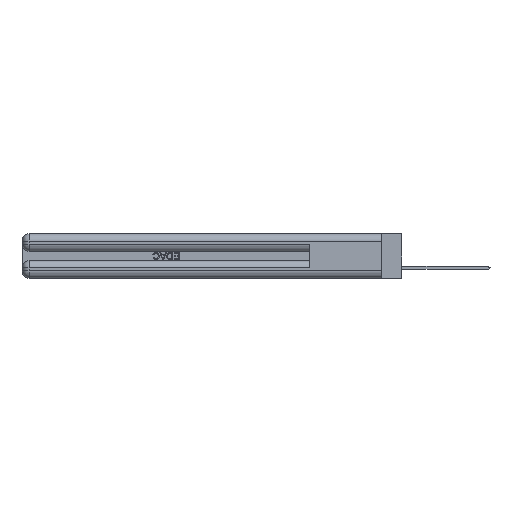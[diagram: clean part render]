
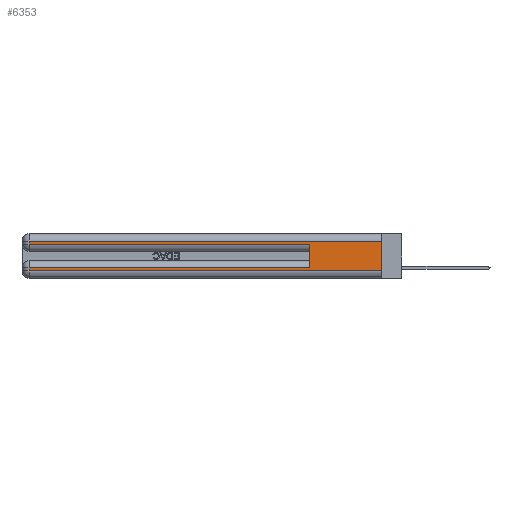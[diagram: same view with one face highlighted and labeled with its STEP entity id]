
A CAD part, left-side view. The second image highlights one B-rep face of the part: STEP entity #6353.
In plain terms, the highlighted planar face has unit normal (-1, 0, 0).
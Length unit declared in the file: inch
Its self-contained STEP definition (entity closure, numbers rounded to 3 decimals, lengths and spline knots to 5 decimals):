
#823 = LINE ( 'NONE', #51536, #43742 ) ;
#1345 = VECTOR ( 'NONE', #28418, 39.37008 ) ;
#1514 = CARTESIAN_POINT ( 'NONE',  ( 0., 0.6, 0.085 ) ) ;
#2061 = AXIS2_PLACEMENT_3D ( 'NONE', #14493, #38792, #19449 ) ;
#2967 = VERTEX_POINT ( 'NONE', #52110 ) ;
#2993 = ORIENTED_EDGE ( 'NONE', *, *, #46046, .T. ) ;
#3393 = CARTESIAN_POINT ( 'NONE',  ( 0., 2.94, 0.37 ) ) ;
#4040 = DIRECTION ( 'NONE',  ( 0., 0., -1. ) ) ;
#4673 = EDGE_LOOP ( 'NONE', ( #17953, #2993, #53097, #30266, #6761, #10194, #51034, #38221 ) ) ;
#4704 = VECTOR ( 'NONE', #52889, 39.37008 ) ;
#4742 = LINE ( 'NONE', #49902, #22289 ) ;
#6000 = DIRECTION ( 'NONE',  ( 0., 1., 0. ) ) ;
#6353 = ADVANCED_FACE ( 'NONE', ( #23500 ), #45315, .F. ) ;
#6634 = VERTEX_POINT ( 'NONE', #34424 ) ;
#6761 = ORIENTED_EDGE ( 'NONE', *, *, #43200, .F. ) ;
#7972 = VECTOR ( 'NONE', #41180, 39.37008 ) ;
#8007 = CARTESIAN_POINT ( 'NONE',  ( 0., 2.94, 0.37 ) ) ;
#8946 = LINE ( 'NONE', #8007, #40845 ) ;
#9210 = CARTESIAN_POINT ( 'NONE',  ( 0., 0., 0.31 ) ) ;
#9835 = EDGE_CURVE ( 'NONE', #46352, #6634, #4742, .T. ) ;
#10194 = ORIENTED_EDGE ( 'NONE', *, *, #9835, .T. ) ;
#10923 = EDGE_CURVE ( 'NONE', #34672, #27907, #16468, .T. ) ;
#14493 = CARTESIAN_POINT ( 'NONE',  ( 0., 0., 0.37 ) ) ;
#15428 = CARTESIAN_POINT ( 'NONE',  ( 0., 0., 0.06 ) ) ;
#16468 = LINE ( 'NONE', #15428, #4704 ) ;
#17696 = VECTOR ( 'NONE', #37283, 39.37008 ) ;
#17953 = ORIENTED_EDGE ( 'NONE', *, *, #19910, .F. ) ;
#19449 = DIRECTION ( 'NONE',  ( 0., 0., -1. ) ) ;
#19910 = EDGE_CURVE ( 'NONE', #45736, #27907, #39017, .T. ) ;
#20435 = CARTESIAN_POINT ( 'NONE',  ( 0., 0., 0.06 ) ) ;
#22289 = VECTOR ( 'NONE', #6000, 39.37008 ) ;
#22754 = DIRECTION ( 'NONE',  ( 0., -1., 0. ) ) ;
#23452 = VECTOR ( 'NONE', #53284, 39.37008 ) ;
#23500 = FACE_OUTER_BOUND ( 'NONE', #4673, .T. ) ;
#23781 = CARTESIAN_POINT ( 'NONE',  ( 0., 0., 0.31 ) ) ;
#24923 = LINE ( 'NONE', #3393, #17696 ) ;
#26024 = LINE ( 'NONE', #23781, #7972 ) ;
#27907 = VERTEX_POINT ( 'NONE', #20435 ) ;
#28418 = DIRECTION ( 'NONE',  ( 0., 0., -1. ) ) ;
#30266 = ORIENTED_EDGE ( 'NONE', *, *, #35251, .T. ) ;
#30889 = EDGE_CURVE ( 'NONE', #39865, #48183, #8946, .T. ) ;
#34424 = CARTESIAN_POINT ( 'NONE',  ( 0., 2.94, 0.085 ) ) ;
#34672 = VERTEX_POINT ( 'NONE', #41636 ) ;
#35251 = EDGE_CURVE ( 'NONE', #48183, #2967, #823, .T. ) ;
#37283 = DIRECTION ( 'NONE',  ( 0., 0., -1. ) ) ;
#38221 = ORIENTED_EDGE ( 'NONE', *, *, #10923, .T. ) ;
#38327 = LINE ( 'NONE', #45005, #23452 ) ;
#38432 = CARTESIAN_POINT ( 'NONE',  ( 0., 0., 0.37 ) ) ;
#38792 = DIRECTION ( 'NONE',  ( 1., 0., 0. ) ) ;
#39017 = LINE ( 'NONE', #38432, #1345 ) ;
#39865 = VERTEX_POINT ( 'NONE', #44626 ) ;
#40845 = VECTOR ( 'NONE', #4040, 39.37008 ) ;
#41180 = DIRECTION ( 'NONE',  ( 0., 1., 0. ) ) ;
#41192 = EDGE_CURVE ( 'NONE', #6634, #34672, #24923, .T. ) ;
#41636 = CARTESIAN_POINT ( 'NONE',  ( 0., 2.94, 0.06 ) ) ;
#41950 = CARTESIAN_POINT ( 'NONE',  ( 0., 2.94, 0.285 ) ) ;
#43200 = EDGE_CURVE ( 'NONE', #46352, #2967, #38327, .T. ) ;
#43742 = VECTOR ( 'NONE', #22754, 39.37008 ) ;
#44626 = CARTESIAN_POINT ( 'NONE',  ( 0., 2.94, 0.31 ) ) ;
#45005 = CARTESIAN_POINT ( 'NONE',  ( 0., 0.6, 0.145 ) ) ;
#45315 = PLANE ( 'NONE',  #2061 ) ;
#45736 = VERTEX_POINT ( 'NONE', #9210 ) ;
#46046 = EDGE_CURVE ( 'NONE', #45736, #39865, #26024, .T. ) ;
#46352 = VERTEX_POINT ( 'NONE', #1514 ) ;
#48183 = VERTEX_POINT ( 'NONE', #41950 ) ;
#49902 = CARTESIAN_POINT ( 'NONE',  ( 0., 0., 0.085 ) ) ;
#51034 = ORIENTED_EDGE ( 'NONE', *, *, #41192, .T. ) ;
#51536 = CARTESIAN_POINT ( 'NONE',  ( 0., 0., 0.285 ) ) ;
#52110 = CARTESIAN_POINT ( 'NONE',  ( 0., 0.6, 0.285 ) ) ;
#52889 = DIRECTION ( 'NONE',  ( 0., -1., 0. ) ) ;
#53097 = ORIENTED_EDGE ( 'NONE', *, *, #30889, .T. ) ;
#53284 = DIRECTION ( 'NONE',  ( 0., 0., 1. ) ) ;
